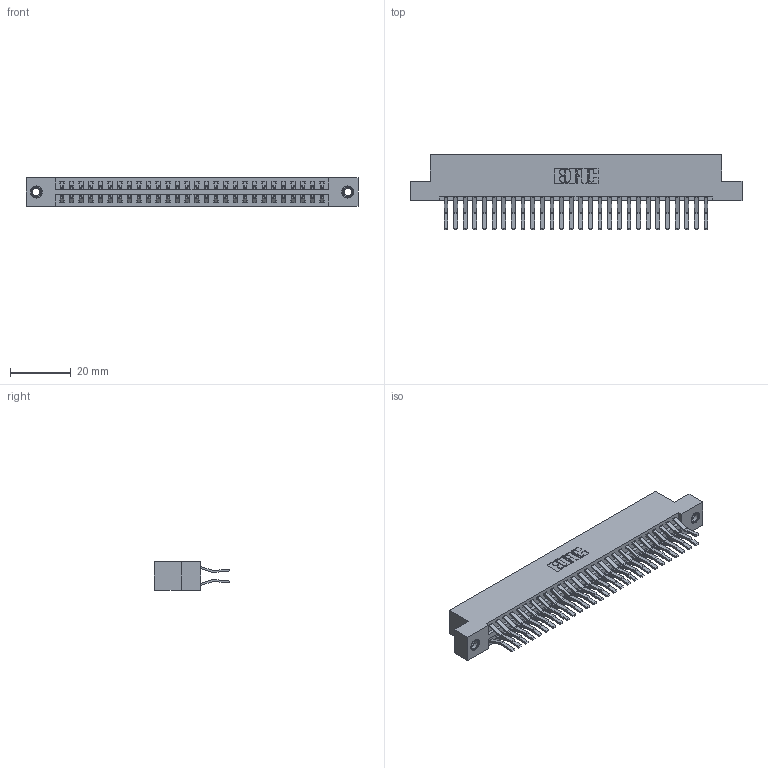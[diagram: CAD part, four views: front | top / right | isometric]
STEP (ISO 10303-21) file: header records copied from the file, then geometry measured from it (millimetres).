
FILE_DESCRIPTION (( 'STEP AP203' ), '1' );
FILE_NAME ('346-056-560-207.STEP', '2022-05-21T07:07:16', ( '' ), ( '' ), 'SwSTEP 2.0', 'SolidWorks 2020', '' );
FILE_SCHEMA (( 'CONFIG_CONTROL_DESIGN' ));
Length unit declared in the file: inch
Products named in the file (4): 345-292-001_560 Tail; 345-250-001_345-250-005-103; 346 Part_Flush Mounting Lugs - 0.156 Dia-TI; 346-056-560-207
Assembly tree (59 placements, depth 2):
  346-056-560-207
    346 Part_Flush Mounting Lugs - 0.156 Dia-TI
    345-292-001_560 Tail  x56
    345-250-001_345-250-005-103  x2
Bounding box: 109.47 x 24.78 x 9.4 mm (x, y, z)
Volume: 10919.9 mm3; surface area: 15803.1 mm2
Topology: 59 solids, 59 shells, 3206 faces, 9481 edges, 6238 vertices
Faces by surface type: plane 2068, cylinder 1122, cone 12, torus 4
Entity records: 21432 total; most frequent: CARTESIAN_POINT 3535, ORIENTED_EDGE 3462, DIRECTION 3197, EDGE_CURVE 1731, VECTOR 1463, LINE 1463, VERTEX_POINT 1148, AXIS2_PLACEMENT_3D 867
